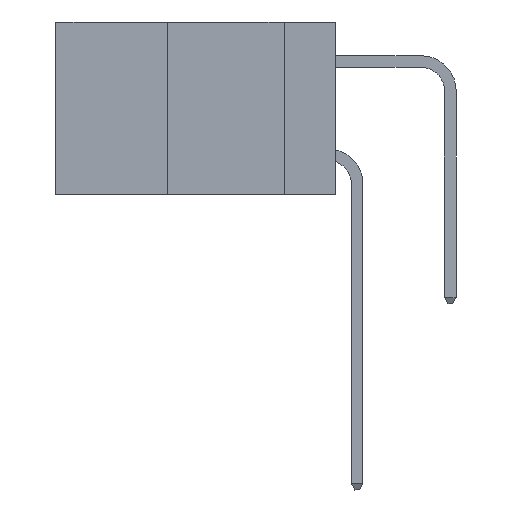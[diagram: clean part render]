
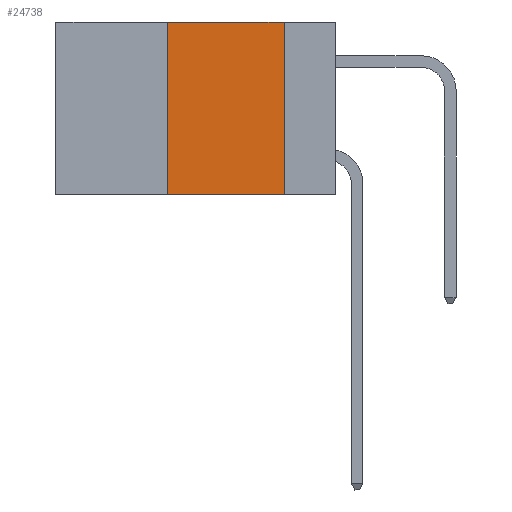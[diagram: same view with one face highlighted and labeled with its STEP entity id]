
A CAD part, left-side view. The second image highlights one B-rep face of the part: STEP entity #24738.
In plain terms, the highlighted planar face has unit normal (-1, 0, 0).
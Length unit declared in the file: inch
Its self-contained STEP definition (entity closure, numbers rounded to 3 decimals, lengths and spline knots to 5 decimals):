
#596 = EDGE_CURVE ( 'NONE', #9055, #10850, #14428, .T. ) ;
#2756 = VERTEX_POINT ( 'NONE', #14383 ) ;
#3557 = CARTESIAN_POINT ( 'NONE',  ( 0., 0.11, 0. ) ) ;
#4074 = CARTESIAN_POINT ( 'NONE',  ( 0., 0.6, 0. ) ) ;
#5845 = LINE ( 'NONE', #11507, #23657 ) ;
#8017 = ORIENTED_EDGE ( 'NONE', *, *, #596, .F. ) ;
#8128 = LINE ( 'NONE', #32449, #19205 ) ;
#9055 = VERTEX_POINT ( 'NONE', #28750 ) ;
#10850 = VERTEX_POINT ( 'NONE', #3557 ) ;
#11175 = ORIENTED_EDGE ( 'NONE', *, *, #21637, .F. ) ;
#11441 = DIRECTION ( 'NONE',  ( 0., 0., -1. ) ) ;
#11507 = CARTESIAN_POINT ( 'NONE',  ( 0., 0.6, -0.37 ) ) ;
#12759 = EDGE_LOOP ( 'NONE', ( #17727, #8017, #11175, #28925 ) ) ;
#12828 = PLANE ( 'NONE',  #27995 ) ;
#13216 = FACE_OUTER_BOUND ( 'NONE', #12759, .T. ) ;
#13439 = CARTESIAN_POINT ( 'NONE',  ( 0., 0.11, -0.37 ) ) ;
#14383 = CARTESIAN_POINT ( 'NONE',  ( 0., 0.36, -0.37 ) ) ;
#14428 = LINE ( 'NONE', #23557, #35099 ) ;
#17727 = ORIENTED_EDGE ( 'NONE', *, *, #35462, .F. ) ;
#19205 = VECTOR ( 'NONE', #28948, 39.37008 ) ;
#19734 = VERTEX_POINT ( 'NONE', #13439 ) ;
#20827 = DIRECTION ( 'NONE',  ( 0., -1., 0. ) ) ;
#21637 = EDGE_CURVE ( 'NONE', #2756, #9055, #8128, .T. ) ;
#22157 = DIRECTION ( 'NONE',  ( 0., 0., -1. ) ) ;
#23341 = DIRECTION ( 'NONE',  ( 0., -1., 0. ) ) ;
#23471 = CARTESIAN_POINT ( 'NONE',  ( 0., 0.11, 0. ) ) ;
#23557 = CARTESIAN_POINT ( 'NONE',  ( 0., 0.6, 0. ) ) ;
#23657 = VECTOR ( 'NONE', #23341, 39.37008 ) ;
#24738 = ADVANCED_FACE ( 'NONE', ( #13216 ), #12828, .F. ) ;
#25080 = DIRECTION ( 'NONE',  ( 1., 0., 0. ) ) ;
#25665 = EDGE_CURVE ( 'NONE', #2756, #19734, #5845, .T. ) ;
#27995 = AXIS2_PLACEMENT_3D ( 'NONE', #4074, #25080, #22157 ) ;
#28750 = CARTESIAN_POINT ( 'NONE',  ( 0., 0.36, 0. ) ) ;
#28925 = ORIENTED_EDGE ( 'NONE', *, *, #25665, .T. ) ;
#28948 = DIRECTION ( 'NONE',  ( 0., 0., 1. ) ) ;
#32449 = CARTESIAN_POINT ( 'NONE',  ( 0., 0.36, 0. ) ) ;
#35099 = VECTOR ( 'NONE', #20827, 39.37008 ) ;
#35462 = EDGE_CURVE ( 'NONE', #10850, #19734, #38103, .T. ) ;
#37108 = VECTOR ( 'NONE', #11441, 39.37008 ) ;
#38103 = LINE ( 'NONE', #23471, #37108 ) ;
